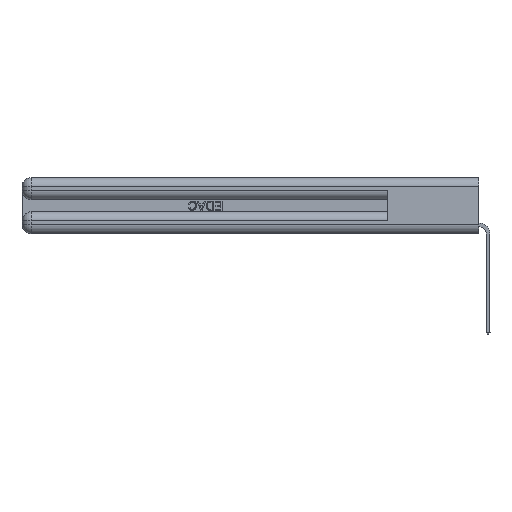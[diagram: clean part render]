
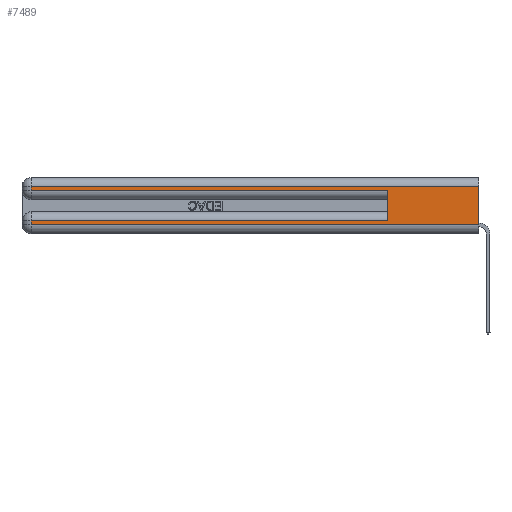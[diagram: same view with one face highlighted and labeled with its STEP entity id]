
A CAD part, left-side view. The second image highlights one B-rep face of the part: STEP entity #7489.
In plain terms, the highlighted planar face has unit normal (-1, 0, 0).
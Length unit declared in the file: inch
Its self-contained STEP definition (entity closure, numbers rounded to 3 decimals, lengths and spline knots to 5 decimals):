
#107 = LINE ( 'NONE', #6801, #11492 ) ;
#289 = CARTESIAN_POINT ( 'NONE',  ( 0., 0., 0.285 ) ) ;
#371 = LINE ( 'NONE', #4057, #15690 ) ;
#524 = DIRECTION ( 'NONE',  ( 0., 0., -1. ) ) ;
#910 = DIRECTION ( 'NONE',  ( 0., 1., 0. ) ) ;
#935 = ORIENTED_EDGE ( 'NONE', *, *, #16295, .T. ) ;
#1017 = DIRECTION ( 'NONE',  ( 0., 1., 0. ) ) ;
#1018 = CARTESIAN_POINT ( 'NONE',  ( 0., 2.94, 0.37 ) ) ;
#1102 = EDGE_CURVE ( 'NONE', #14094, #24741, #15354, .T. ) ;
#1360 = DIRECTION ( 'NONE',  ( 0., 0., -1. ) ) ;
#1464 = ORIENTED_EDGE ( 'NONE', *, *, #3800, .T. ) ;
#2142 = VECTOR ( 'NONE', #6310, 39.37008 ) ;
#2699 = EDGE_CURVE ( 'NONE', #6602, #16594, #8469, .T. ) ;
#3323 = CARTESIAN_POINT ( 'NONE',  ( 0., 0., 0.31 ) ) ;
#3800 = EDGE_CURVE ( 'NONE', #18727, #7240, #371, .T. ) ;
#3877 = EDGE_LOOP ( 'NONE', ( #22638, #935, #20608, #9122, #24291, #10278, #21713, #1464 ) ) ;
#4057 = CARTESIAN_POINT ( 'NONE',  ( 0., 0., 0.06 ) ) ;
#5574 = VECTOR ( 'NONE', #9325, 39.37008 ) ;
#5677 = EDGE_CURVE ( 'NONE', #21728, #7240, #20048, .T. ) ;
#6310 = DIRECTION ( 'NONE',  ( 0., -1., 0. ) ) ;
#6602 = VERTEX_POINT ( 'NONE', #8712 ) ;
#6626 = VECTOR ( 'NONE', #1360, 39.37008 ) ;
#6801 = CARTESIAN_POINT ( 'NONE',  ( 0., 2.94, 0.37 ) ) ;
#7240 = VERTEX_POINT ( 'NONE', #25830 ) ;
#7489 = ADVANCED_FACE ( 'NONE', ( #14801 ), #8792, .F. ) ;
#7683 = LINE ( 'NONE', #3323, #12854 ) ;
#8469 = LINE ( 'NONE', #289, #2142 ) ;
#8503 = DIRECTION ( 'NONE',  ( 1., 0., 0. ) ) ;
#8712 = CARTESIAN_POINT ( 'NONE',  ( 0., 2.94, 0.285 ) ) ;
#8792 = PLANE ( 'NONE',  #20838 ) ;
#8871 = VECTOR ( 'NONE', #910, 39.37008 ) ;
#8885 = CARTESIAN_POINT ( 'NONE',  ( 0., 0.6, 0.285 ) ) ;
#9122 = ORIENTED_EDGE ( 'NONE', *, *, #2699, .T. ) ;
#9325 = DIRECTION ( 'NONE',  ( 0., 0., -1. ) ) ;
#10278 = ORIENTED_EDGE ( 'NONE', *, *, #1102, .T. ) ;
#10814 = CARTESIAN_POINT ( 'NONE',  ( 0., 2.94, 0.06 ) ) ;
#11290 = CARTESIAN_POINT ( 'NONE',  ( 0., 2.94, 0.31 ) ) ;
#11395 = LINE ( 'NONE', #1018, #5574 ) ;
#11492 = VECTOR ( 'NONE', #524, 39.37008 ) ;
#11848 = CARTESIAN_POINT ( 'NONE',  ( 0., 0., 0.37 ) ) ;
#12854 = VECTOR ( 'NONE', #1017, 39.37008 ) ;
#14094 = VERTEX_POINT ( 'NONE', #17848 ) ;
#14567 = DIRECTION ( 'NONE',  ( 0., -1., 0. ) ) ;
#14801 = FACE_OUTER_BOUND ( 'NONE', #3877, .T. ) ;
#14931 = CARTESIAN_POINT ( 'NONE',  ( 0., 0., 0.37 ) ) ;
#15354 = LINE ( 'NONE', #15625, #8871 ) ;
#15625 = CARTESIAN_POINT ( 'NONE',  ( 0., 0., 0.085 ) ) ;
#15690 = VECTOR ( 'NONE', #14567, 39.37008 ) ;
#16295 = EDGE_CURVE ( 'NONE', #21728, #16899, #7683, .T. ) ;
#16551 = DIRECTION ( 'NONE',  ( 0., 0., -1. ) ) ;
#16594 = VERTEX_POINT ( 'NONE', #8885 ) ;
#16899 = VERTEX_POINT ( 'NONE', #11290 ) ;
#17848 = CARTESIAN_POINT ( 'NONE',  ( 0., 0.6, 0.085 ) ) ;
#18171 = VECTOR ( 'NONE', #18971, 39.37008 ) ;
#18494 = CARTESIAN_POINT ( 'NONE',  ( 0., 2.94, 0.085 ) ) ;
#18727 = VERTEX_POINT ( 'NONE', #10814 ) ;
#18971 = DIRECTION ( 'NONE',  ( 0., 0., 1. ) ) ;
#19257 = CARTESIAN_POINT ( 'NONE',  ( 0., 0.6, 0.145 ) ) ;
#20009 = CARTESIAN_POINT ( 'NONE',  ( 0., 0., 0.31 ) ) ;
#20048 = LINE ( 'NONE', #11848, #6626 ) ;
#20608 = ORIENTED_EDGE ( 'NONE', *, *, #22067, .T. ) ;
#20665 = EDGE_CURVE ( 'NONE', #24741, #18727, #107, .T. ) ;
#20838 = AXIS2_PLACEMENT_3D ( 'NONE', #14931, #8503, #16551 ) ;
#21182 = EDGE_CURVE ( 'NONE', #14094, #16594, #25339, .T. ) ;
#21713 = ORIENTED_EDGE ( 'NONE', *, *, #20665, .T. ) ;
#21728 = VERTEX_POINT ( 'NONE', #20009 ) ;
#22067 = EDGE_CURVE ( 'NONE', #16899, #6602, #11395, .T. ) ;
#22638 = ORIENTED_EDGE ( 'NONE', *, *, #5677, .F. ) ;
#24291 = ORIENTED_EDGE ( 'NONE', *, *, #21182, .F. ) ;
#24741 = VERTEX_POINT ( 'NONE', #18494 ) ;
#25339 = LINE ( 'NONE', #19257, #18171 ) ;
#25830 = CARTESIAN_POINT ( 'NONE',  ( 0., 0., 0.06 ) ) ;
